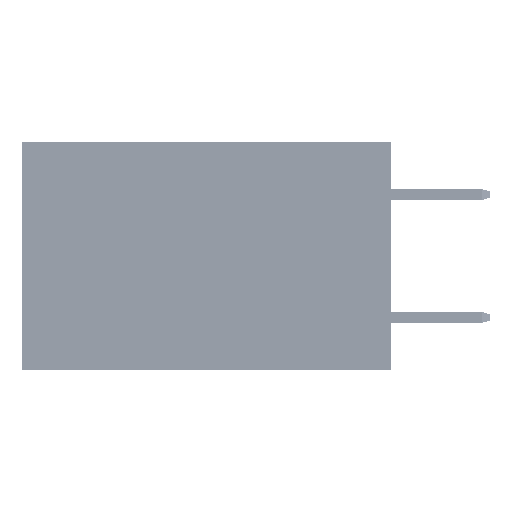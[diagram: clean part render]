
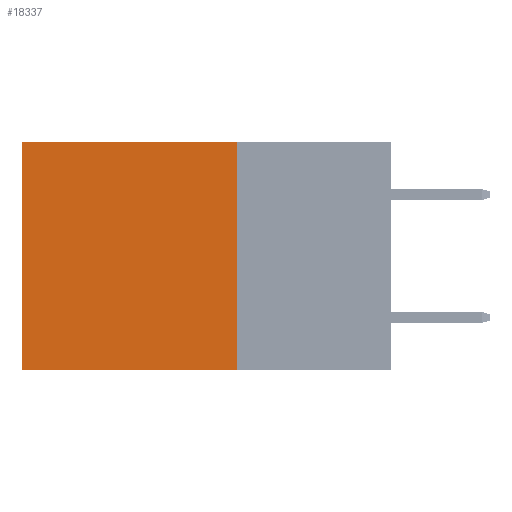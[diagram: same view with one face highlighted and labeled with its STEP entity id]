
A CAD part, left-side view. The second image highlights one B-rep face of the part: STEP entity #18337.
In plain terms, the highlighted planar face has unit normal (-1, 0, 0).
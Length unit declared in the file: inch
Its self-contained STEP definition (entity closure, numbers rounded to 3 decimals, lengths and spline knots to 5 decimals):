
#323 = CARTESIAN_POINT ( 'NONE',  ( 0.2875, 0.25, -0.37 ) ) ;
#2406 = VERTEX_POINT ( 'NONE', #23194 ) ;
#3036 = VECTOR ( 'NONE', #29061, 39.37008 ) ;
#3686 = LINE ( 'NONE', #323, #29440 ) ;
#8468 = CARTESIAN_POINT ( 'NONE',  ( 0.2875, 0.25, 0. ) ) ;
#8535 = CARTESIAN_POINT ( 'NONE',  ( 0.2875, 0.25, 0. ) ) ;
#8563 = PLANE ( 'NONE',  #28492 ) ;
#9952 = LINE ( 'NONE', #41483, #3036 ) ;
#14074 = CARTESIAN_POINT ( 'NONE',  ( 0.2875, 0.25, 0. ) ) ;
#15315 = CARTESIAN_POINT ( 'NONE',  ( 0.2875, 0.25, -0.37 ) ) ;
#18239 = VERTEX_POINT ( 'NONE', #15315 ) ;
#18337 = ADVANCED_FACE ( 'NONE', ( #24064 ), #8563, .F. ) ;
#18706 = DIRECTION ( 'NONE',  ( 0., 1., 0. ) ) ;
#22398 = EDGE_CURVE ( 'NONE', #2406, #32548, #9952, .T. ) ;
#23181 = EDGE_CURVE ( 'NONE', #18239, #32548, #3686, .T. ) ;
#23194 = CARTESIAN_POINT ( 'NONE',  ( 0.2875, 0.6, 0. ) ) ;
#24064 = FACE_OUTER_BOUND ( 'NONE', #38457, .T. ) ;
#24283 = ORIENTED_EDGE ( 'NONE', *, *, #23181, .F. ) ;
#24312 = CARTESIAN_POINT ( 'NONE',  ( 0.2875, 0.25, 0. ) ) ;
#25428 = LINE ( 'NONE', #14074, #33450 ) ;
#28492 = AXIS2_PLACEMENT_3D ( 'NONE', #24312, #43467, #39577 ) ;
#29061 = DIRECTION ( 'NONE',  ( 0., 0., -1. ) ) ;
#29219 = ORIENTED_EDGE ( 'NONE', *, *, #35917, .T. ) ;
#29440 = VECTOR ( 'NONE', #42947, 39.37008 ) ;
#31012 = DIRECTION ( 'NONE',  ( 0., 0., -1. ) ) ;
#31075 = EDGE_CURVE ( 'NONE', #39684, #18239, #47799, .T. ) ;
#32548 = VERTEX_POINT ( 'NONE', #47612 ) ;
#33450 = VECTOR ( 'NONE', #18706, 39.37008 ) ;
#35615 = ORIENTED_EDGE ( 'NONE', *, *, #31075, .F. ) ;
#35917 = EDGE_CURVE ( 'NONE', #39684, #2406, #25428, .T. ) ;
#38457 = EDGE_LOOP ( 'NONE', ( #49618, #24283, #35615, #29219 ) ) ;
#39577 = DIRECTION ( 'NONE',  ( 0., 0., -1. ) ) ;
#39684 = VERTEX_POINT ( 'NONE', #8468 ) ;
#41483 = CARTESIAN_POINT ( 'NONE',  ( 0.2875, 0.6, 0. ) ) ;
#42947 = DIRECTION ( 'NONE',  ( 0., 1., 0. ) ) ;
#43467 = DIRECTION ( 'NONE',  ( 1., 0., 0. ) ) ;
#47257 = VECTOR ( 'NONE', #31012, 39.37008 ) ;
#47612 = CARTESIAN_POINT ( 'NONE',  ( 0.2875, 0.6, -0.37 ) ) ;
#47799 = LINE ( 'NONE', #8535, #47257 ) ;
#49618 = ORIENTED_EDGE ( 'NONE', *, *, #22398, .T. ) ;
